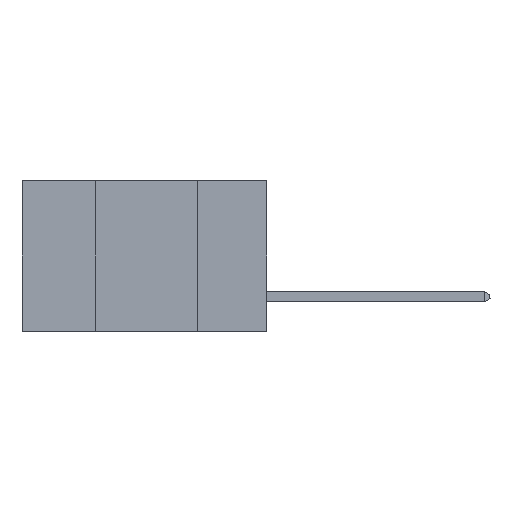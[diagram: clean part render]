
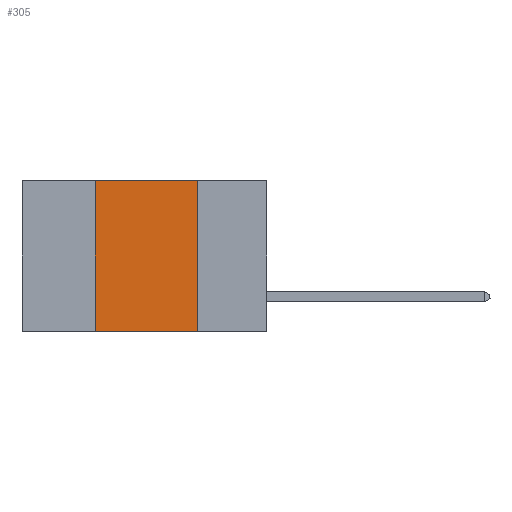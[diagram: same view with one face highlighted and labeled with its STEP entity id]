
A CAD part, left-side view. The second image highlights one B-rep face of the part: STEP entity #305.
In plain terms, the highlighted planar face has unit normal (-1, 0, 0).
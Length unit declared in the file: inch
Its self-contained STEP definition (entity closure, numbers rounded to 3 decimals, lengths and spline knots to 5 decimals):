
#163 = DIRECTION ( 'NONE',  ( 0., -1., 0. ) ) ;
#182 = VERTEX_POINT ( 'NONE', #1842 ) ;
#305 = ADVANCED_FACE ( 'NONE', ( #9755 ), #5527, .F. ) ;
#680 = DIRECTION ( 'NONE',  ( 0., -1., 0. ) ) ;
#1489 = ORIENTED_EDGE ( 'NONE', *, *, #6779, .T. ) ;
#1531 = ORIENTED_EDGE ( 'NONE', *, *, #1598, .F. ) ;
#1554 = EDGE_CURVE ( 'NONE', #5957, #6719, #9001, .T. ) ;
#1598 = EDGE_CURVE ( 'NONE', #9961, #5957, #6897, .T. ) ;
#1714 = CARTESIAN_POINT ( 'NONE',  ( 0., 0.42, 0. ) ) ;
#1842 = CARTESIAN_POINT ( 'NONE',  ( 0., 0.42, -0.37 ) ) ;
#1922 = LINE ( 'NONE', #1714, #5040 ) ;
#2054 = EDGE_LOOP ( 'NONE', ( #5806, #1531, #9811, #1489 ) ) ;
#2874 = CARTESIAN_POINT ( 'NONE',  ( 0., 0.6, 0. ) ) ;
#3013 = DIRECTION ( 'NONE',  ( 0., 0., -1. ) ) ;
#3584 = LINE ( 'NONE', #6166, #10895 ) ;
#5040 = VECTOR ( 'NONE', #6803, 39.37008 ) ;
#5527 = PLANE ( 'NONE',  #10045 ) ;
#5801 = VECTOR ( 'NONE', #680, 39.37008 ) ;
#5806 = ORIENTED_EDGE ( 'NONE', *, *, #1554, .F. ) ;
#5957 = VERTEX_POINT ( 'NONE', #6239 ) ;
#5979 = CARTESIAN_POINT ( 'NONE',  ( 0., 0.6, 0. ) ) ;
#6166 = CARTESIAN_POINT ( 'NONE',  ( 0., 0.6, -0.37 ) ) ;
#6239 = CARTESIAN_POINT ( 'NONE',  ( 0., 0.17, 0. ) ) ;
#6368 = DIRECTION ( 'NONE',  ( 1., 0., 0. ) ) ;
#6719 = VERTEX_POINT ( 'NONE', #7831 ) ;
#6779 = EDGE_CURVE ( 'NONE', #182, #6719, #3584, .T. ) ;
#6803 = DIRECTION ( 'NONE',  ( 0., 0., 1. ) ) ;
#6869 = CARTESIAN_POINT ( 'NONE',  ( 0., 0.17, 0. ) ) ;
#6897 = LINE ( 'NONE', #5979, #5801 ) ;
#7831 = CARTESIAN_POINT ( 'NONE',  ( 0., 0.17, -0.37 ) ) ;
#8163 = VECTOR ( 'NONE', #11268, 39.37008 ) ;
#9001 = LINE ( 'NONE', #6869, #8163 ) ;
#9013 = EDGE_CURVE ( 'NONE', #182, #9961, #1922, .T. ) ;
#9088 = CARTESIAN_POINT ( 'NONE',  ( 0., 0.42, 0. ) ) ;
#9755 = FACE_OUTER_BOUND ( 'NONE', #2054, .T. ) ;
#9811 = ORIENTED_EDGE ( 'NONE', *, *, #9013, .F. ) ;
#9961 = VERTEX_POINT ( 'NONE', #9088 ) ;
#10045 = AXIS2_PLACEMENT_3D ( 'NONE', #2874, #6368, #3013 ) ;
#10895 = VECTOR ( 'NONE', #163, 39.37008 ) ;
#11268 = DIRECTION ( 'NONE',  ( 0., 0., -1. ) ) ;
